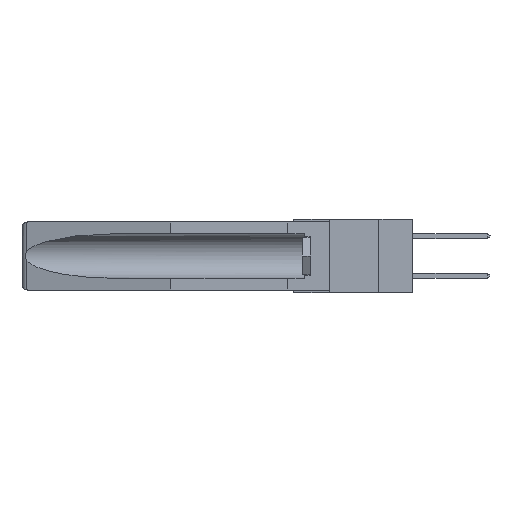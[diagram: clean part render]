
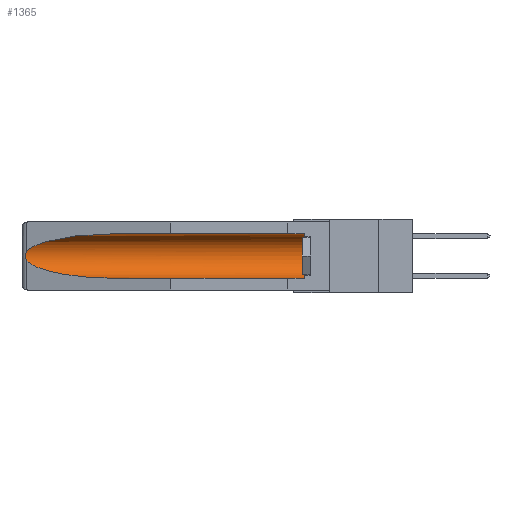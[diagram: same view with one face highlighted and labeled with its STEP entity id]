
A CAD part, left-side view. The second image highlights one B-rep face of the part: STEP entity #1365.
In plain terms, the highlighted cylindrical face has radius 2.857 mm (diameter 5.715 mm), a partial arc.
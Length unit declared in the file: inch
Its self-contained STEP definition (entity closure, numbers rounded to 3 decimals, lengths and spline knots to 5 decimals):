
#277 = CARTESIAN_POINT ( 'NONE',  ( 0.26537, 1.52718, -0.14972 ) ) ;
#567 = CYLINDRICAL_SURFACE ( 'NONE', #17128, 0.1125 ) ;
#730 = CARTESIAN_POINT ( 'NONE',  ( 0.26537, 1.52718, -0.14972 ) ) ;
#1118 = CARTESIAN_POINT ( 'NONE',  ( 0.155, -0.30754, -0.1715 ) ) ;
#1365 = ADVANCED_FACE ( 'NONE', ( #1953 ), #567, .F. ) ;
#1906 =( BOUNDED_CURVE ( )  B_SPLINE_CURVE ( 3, ( #20210, #2043, #22516, #730 ),
 .UNSPECIFIED., .F., .F. ) 
 B_SPLINE_CURVE_WITH_KNOTS ( ( 4, 4 ),
 ( 4.71239, 6.08839 ),
 .UNSPECIFIED. ) 
 CURVE ( )  GEOMETRIC_REPRESENTATION_ITEM ( )  RATIONAL_B_SPLINE_CURVE ( ( 1., 0.848, 0.848, 1. ) ) 
 REPRESENTATION_ITEM ( '' )  );
#1953 = FACE_OUTER_BOUND ( 'NONE', #12780, .T. ) ;
#2043 = CARTESIAN_POINT ( 'NONE',  ( 0.21114, 1.30732, -0.059 ) ) ;
#2103 = VERTEX_POINT ( 'NONE', #18094 ) ;
#2606 = VERTEX_POINT ( 'NONE', #8889 ) ;
#2816 = CARTESIAN_POINT ( 'NONE',  ( 0.21114, 1.30732, -0.284 ) ) ;
#3353 = CARTESIAN_POINT ( 'NONE',  ( 0.155, 0.126, -0.1715 ) ) ;
#3425 = DIRECTION ( 'NONE',  ( 0., 0., 1. ) ) ;
#4085 = CARTESIAN_POINT ( 'NONE',  ( 0.26597, 1.52961, -0.15275 ) ) ;
#4172 = CARTESIAN_POINT ( 'NONE',  ( 0.26655, 1.53094, -0.18657 ) ) ;
#4811 = AXIS2_PLACEMENT_3D ( 'NONE', #3353, #10463, #3425 ) ;
#4855 = VECTOR ( 'NONE', #12319, 39.37008 ) ;
#4996 = CARTESIAN_POINT ( 'NONE',  ( 0.155, -0.30754, -0.059 ) ) ;
#5012 = DIRECTION ( 'NONE',  ( 0., 0., 1. ) ) ;
#5379 = ORIENTED_EDGE ( 'NONE', *, *, #14345, .T. ) ;
#5911 = CARTESIAN_POINT ( 'NONE',  ( 0.26654, 1.53092, -0.15636 ) ) ;
#5984 = CARTESIAN_POINT ( 'NONE',  ( 0.26537, 1.52718, -0.19328 ) ) ;
#6053 = CARTESIAN_POINT ( 'NONE',  ( 0.2675, 1.53308, -0.16763 ) ) ;
#6598 = DIRECTION ( 'NONE',  ( 0., 1., 0. ) ) ;
#6858 = EDGE_CURVE ( 'NONE', #2606, #7972, #1906, .T. ) ;
#7708 = CARTESIAN_POINT ( 'NONE',  ( 0.2675, 1.53308, -0.17534 ) ) ;
#7904 = EDGE_CURVE ( 'NONE', #20653, #2103, #18748, .T. ) ;
#7972 = VERTEX_POINT ( 'NONE', #23184 ) ;
#8196 = B_SPLINE_CURVE_WITH_KNOTS ( 'NONE', 3,
 ( #277, #4085, #5911, #18667, #6053, #7708, #11408, #4172, #16885, #5984 ),
 .UNSPECIFIED., .F., .F.,
 ( 4, 2, 2, 2, 4 ),
 ( 0., 0.00029, 0.00058, 0.00087, 0.00117 ),
 .UNSPECIFIED. ) ;
#8497 = VERTEX_POINT ( 'NONE', #15039 ) ;
#8889 = CARTESIAN_POINT ( 'NONE',  ( 0.155, 1.07973, -0.059 ) ) ;
#9033 = VECTOR ( 'NONE', #6598, 39.37008 ) ;
#9629 = CIRCLE ( 'NONE', #4811, 0.1125 ) ;
#10165 = CARTESIAN_POINT ( 'NONE',  ( 0.155, 1.07973, -0.284 ) ) ;
#10369 = VERTEX_POINT ( 'NONE', #21364 ) ;
#10445 = DIRECTION ( 'NONE',  ( 0., 1., 0. ) ) ;
#10463 = DIRECTION ( 'NONE',  ( 0., -1., 0. ) ) ;
#10917 = CARTESIAN_POINT ( 'NONE',  ( 0.155, 0.126, -0.284 ) ) ;
#11408 = CARTESIAN_POINT ( 'NONE',  ( 0.2673, 1.53269, -0.17917 ) ) ;
#12263 = LINE ( 'NONE', #4996, #4855 ) ;
#12319 = DIRECTION ( 'NONE',  ( 0., 1., 0. ) ) ;
#12780 = EDGE_LOOP ( 'NONE', ( #17374, #5379, #16877, #19650, #17357, #16420 ) ) ;
#14345 = EDGE_CURVE ( 'NONE', #7972, #8497, #8196, .T. ) ;
#14882 = EDGE_CURVE ( 'NONE', #10369, #2606, #12263, .T. ) ;
#15039 = CARTESIAN_POINT ( 'NONE',  ( 0.26537, 1.52718, -0.19328 ) ) ;
#16025 = EDGE_CURVE ( 'NONE', #20653, #10369, #9629, .T. ) ;
#16420 = ORIENTED_EDGE ( 'NONE', *, *, #14882, .T. ) ;
#16877 = ORIENTED_EDGE ( 'NONE', *, *, #18387, .T. ) ;
#16885 = CARTESIAN_POINT ( 'NONE',  ( 0.26597, 1.5296, -0.19026 ) ) ;
#17128 = AXIS2_PLACEMENT_3D ( 'NONE', #1118, #10445, #5012 ) ;
#17357 = ORIENTED_EDGE ( 'NONE', *, *, #16025, .T. ) ;
#17374 = ORIENTED_EDGE ( 'NONE', *, *, #6858, .T. ) ;
#17387 = CARTESIAN_POINT ( 'NONE',  ( 0.26537, 1.52718, -0.19328 ) ) ;
#17535 = CARTESIAN_POINT ( 'NONE',  ( 0.155, -0.30754, -0.284 ) ) ;
#18094 = CARTESIAN_POINT ( 'NONE',  ( 0.155, 1.07973, -0.284 ) ) ;
#18387 = EDGE_CURVE ( 'NONE', #8497, #2103, #21366, .T. ) ;
#18667 = CARTESIAN_POINT ( 'NONE',  ( 0.2673, 1.5327, -0.16383 ) ) ;
#18748 = LINE ( 'NONE', #17535, #9033 ) ;
#19650 = ORIENTED_EDGE ( 'NONE', *, *, #7904, .F. ) ;
#20210 = CARTESIAN_POINT ( 'NONE',  ( 0.155, 1.07973, -0.059 ) ) ;
#20653 = VERTEX_POINT ( 'NONE', #10917 ) ;
#21075 = CARTESIAN_POINT ( 'NONE',  ( 0.25451, 1.48313, -0.24835 ) ) ;
#21364 = CARTESIAN_POINT ( 'NONE',  ( 0.155, 0.126, -0.059 ) ) ;
#21366 =( BOUNDED_CURVE ( )  B_SPLINE_CURVE ( 3, ( #17387, #21075, #2816, #10165 ),
 .UNSPECIFIED., .F., .F. ) 
 B_SPLINE_CURVE_WITH_KNOTS ( ( 4, 4 ),
 ( 0.1948, 1.5708 ),
 .UNSPECIFIED. ) 
 CURVE ( )  GEOMETRIC_REPRESENTATION_ITEM ( )  RATIONAL_B_SPLINE_CURVE ( ( 1., 0.848, 0.848, 1. ) ) 
 REPRESENTATION_ITEM ( '' )  );
#22516 = CARTESIAN_POINT ( 'NONE',  ( 0.25451, 1.48313, -0.09465 ) ) ;
#23184 = CARTESIAN_POINT ( 'NONE',  ( 0.26537, 1.52718, -0.14972 ) ) ;
